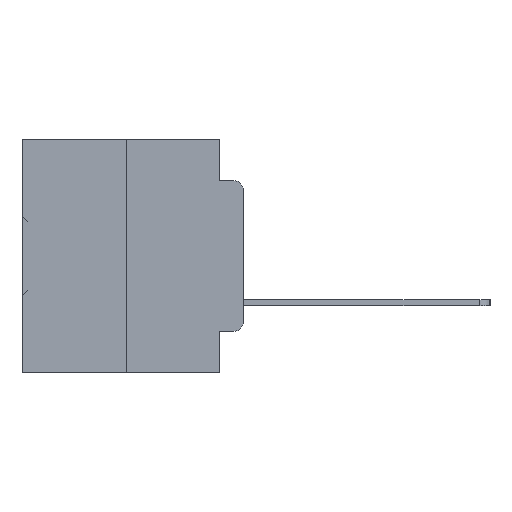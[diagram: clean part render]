
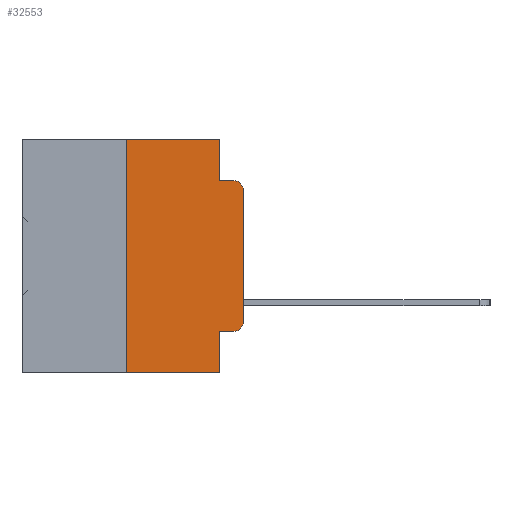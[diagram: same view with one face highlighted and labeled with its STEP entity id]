
A CAD part, left-side view. The second image highlights one B-rep face of the part: STEP entity #32553.
In plain terms, the highlighted planar face has unit normal (-1, 0, 0).
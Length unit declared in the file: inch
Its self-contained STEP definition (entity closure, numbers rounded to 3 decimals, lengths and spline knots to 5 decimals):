
#42 = LINE ( 'NONE', #34371, #6103 ) ;
#466 = VECTOR ( 'NONE', #25881, 39.37008 ) ;
#471 = VERTEX_POINT ( 'NONE', #4795 ) ;
#617 = ORIENTED_EDGE ( 'NONE', *, *, #7409, .T. ) ;
#859 = DIRECTION ( 'NONE',  ( -1., 0., 0. ) ) ;
#871 = EDGE_CURVE ( 'NONE', #471, #37231, #8077, .T. ) ;
#937 = ORIENTED_EDGE ( 'NONE', *, *, #17577, .T. ) ;
#1311 = VERTEX_POINT ( 'NONE', #2736 ) ;
#1438 = LINE ( 'NONE', #36965, #16352 ) ;
#1925 = ORIENTED_EDGE ( 'NONE', *, *, #2875, .T. ) ;
#2629 = DIRECTION ( 'NONE',  ( 0., -1., 0. ) ) ;
#2736 = CARTESIAN_POINT ( 'NONE',  ( 0., 0.051, 0. ) ) ;
#2875 = EDGE_CURVE ( 'NONE', #32249, #471, #1438, .T. ) ;
#3831 = LINE ( 'NONE', #8816, #34455 ) ;
#4253 = CARTESIAN_POINT ( 'NONE',  ( 0., 0.02, -0.4115 ) ) ;
#4795 = CARTESIAN_POINT ( 'NONE',  ( 0., 0., -0.1085 ) ) ;
#6103 = VECTOR ( 'NONE', #16642, 39.37008 ) ;
#6384 = LINE ( 'NONE', #17465, #7327 ) ;
#6673 = PLANE ( 'NONE',  #30578 ) ;
#6678 = CARTESIAN_POINT ( 'NONE',  ( 0., 0.25, 0. ) ) ;
#7107 = AXIS2_PLACEMENT_3D ( 'NONE', #18678, #859, #21670 ) ;
#7261 = ORIENTED_EDGE ( 'NONE', *, *, #17119, .F. ) ;
#7327 = VECTOR ( 'NONE', #2629, 39.37008 ) ;
#7409 = EDGE_CURVE ( 'NONE', #9723, #28805, #8439, .T. ) ;
#7744 = FACE_OUTER_BOUND ( 'NONE', #18145, .T. ) ;
#7934 = DIRECTION ( 'NONE',  ( 0., 0., -1. ) ) ;
#8077 = CIRCLE ( 'NONE', #27322, 0.02 ) ;
#8439 = LINE ( 'NONE', #14013, #466 ) ;
#8816 = CARTESIAN_POINT ( 'NONE',  ( 0., 0.051, 0. ) ) ;
#9723 = VERTEX_POINT ( 'NONE', #17847 ) ;
#10354 = ORIENTED_EDGE ( 'NONE', *, *, #29496, .F. ) ;
#10526 = VECTOR ( 'NONE', #7934, 39.37008 ) ;
#10807 = ORIENTED_EDGE ( 'NONE', *, *, #33447, .F. ) ;
#11574 = ORIENTED_EDGE ( 'NONE', *, *, #25500, .F. ) ;
#11652 = VERTEX_POINT ( 'NONE', #6678 ) ;
#12092 = VECTOR ( 'NONE', #15865, 39.37008 ) ;
#12721 = CARTESIAN_POINT ( 'NONE',  ( 0., 0.02, -0.1085 ) ) ;
#13791 = CARTESIAN_POINT ( 'NONE',  ( 0., 0.051, -0.0885 ) ) ;
#14013 = CARTESIAN_POINT ( 'NONE',  ( 0., 0.473, -0.5 ) ) ;
#15630 = DIRECTION ( 'NONE',  ( 1., 0., 0. ) ) ;
#15661 = DIRECTION ( 'NONE',  ( 0., 0., -1. ) ) ;
#15865 = DIRECTION ( 'NONE',  ( 0., 0., 1. ) ) ;
#16352 = VECTOR ( 'NONE', #19255, 39.37008 ) ;
#16356 = CARTESIAN_POINT ( 'NONE',  ( 0., 0.02, -0.0885 ) ) ;
#16642 = DIRECTION ( 'NONE',  ( 0., -1., 0. ) ) ;
#17119 = EDGE_CURVE ( 'NONE', #11652, #1311, #42, .T. ) ;
#17465 = CARTESIAN_POINT ( 'NONE',  ( 0., 0.051, -0.4115 ) ) ;
#17577 = EDGE_CURVE ( 'NONE', #37163, #32249, #30663, .T. ) ;
#17847 = CARTESIAN_POINT ( 'NONE',  ( 0., 0.25, -0.5 ) ) ;
#18145 = EDGE_LOOP ( 'NONE', ( #1925, #36603, #10807, #10354, #7261, #32350, #617, #11574, #30756, #937 ) ) ;
#18678 = CARTESIAN_POINT ( 'NONE',  ( 0., 0.02, -0.3915 ) ) ;
#19255 = DIRECTION ( 'NONE',  ( 0., 0., 1. ) ) ;
#19545 = EDGE_CURVE ( 'NONE', #27488, #37163, #6384, .T. ) ;
#19932 = LINE ( 'NONE', #24664, #12092 ) ;
#21581 = CARTESIAN_POINT ( 'NONE',  ( 0., 0.051, -0.4115 ) ) ;
#21670 = DIRECTION ( 'NONE',  ( 0., 0., -1. ) ) ;
#22398 = CARTESIAN_POINT ( 'NONE',  ( 0., 0.051, -0.5 ) ) ;
#22514 = VECTOR ( 'NONE', #23214, 39.37008 ) ;
#23214 = DIRECTION ( 'NONE',  ( 0., -1., 0. ) ) ;
#23431 = LINE ( 'NONE', #32001, #22514 ) ;
#24664 = CARTESIAN_POINT ( 'NONE',  ( 0., 0.25, 0. ) ) ;
#25500 = EDGE_CURVE ( 'NONE', #27488, #28805, #3831, .T. ) ;
#25881 = DIRECTION ( 'NONE',  ( 0., -1., 0. ) ) ;
#27028 = CARTESIAN_POINT ( 'NONE',  ( 0., 0., -0.3915 ) ) ;
#27322 = AXIS2_PLACEMENT_3D ( 'NONE', #12721, #33391, #15661 ) ;
#27488 = VERTEX_POINT ( 'NONE', #21581 ) ;
#27499 = EDGE_CURVE ( 'NONE', #9723, #11652, #19932, .T. ) ;
#28805 = VERTEX_POINT ( 'NONE', #22398 ) ;
#29496 = EDGE_CURVE ( 'NONE', #1311, #31235, #34126, .T. ) ;
#30578 = AXIS2_PLACEMENT_3D ( 'NONE', #36189, #15630, #36316 ) ;
#30663 = CIRCLE ( 'NONE', #7107, 0.02 ) ;
#30756 = ORIENTED_EDGE ( 'NONE', *, *, #19545, .T. ) ;
#31235 = VERTEX_POINT ( 'NONE', #13791 ) ;
#31611 = CARTESIAN_POINT ( 'NONE',  ( 0., 0.051, 0. ) ) ;
#32001 = CARTESIAN_POINT ( 'NONE',  ( 0., 0.051, -0.0885 ) ) ;
#32249 = VERTEX_POINT ( 'NONE', #27028 ) ;
#32350 = ORIENTED_EDGE ( 'NONE', *, *, #27499, .F. ) ;
#32553 = ADVANCED_FACE ( 'NONE', ( #7744 ), #6673, .F. ) ;
#33391 = DIRECTION ( 'NONE',  ( -1., 0., 0. ) ) ;
#33447 = EDGE_CURVE ( 'NONE', #31235, #37231, #23431, .T. ) ;
#34126 = LINE ( 'NONE', #31611, #10526 ) ;
#34371 = CARTESIAN_POINT ( 'NONE',  ( 0., 0.473, 0. ) ) ;
#34455 = VECTOR ( 'NONE', #35442, 39.37008 ) ;
#35442 = DIRECTION ( 'NONE',  ( 0., 0., -1. ) ) ;
#36189 = CARTESIAN_POINT ( 'NONE',  ( 0., 0.473, 0. ) ) ;
#36316 = DIRECTION ( 'NONE',  ( 0., 0., -1. ) ) ;
#36603 = ORIENTED_EDGE ( 'NONE', *, *, #871, .T. ) ;
#36965 = CARTESIAN_POINT ( 'NONE',  ( 0., 0., 0. ) ) ;
#37163 = VERTEX_POINT ( 'NONE', #4253 ) ;
#37231 = VERTEX_POINT ( 'NONE', #16356 ) ;
